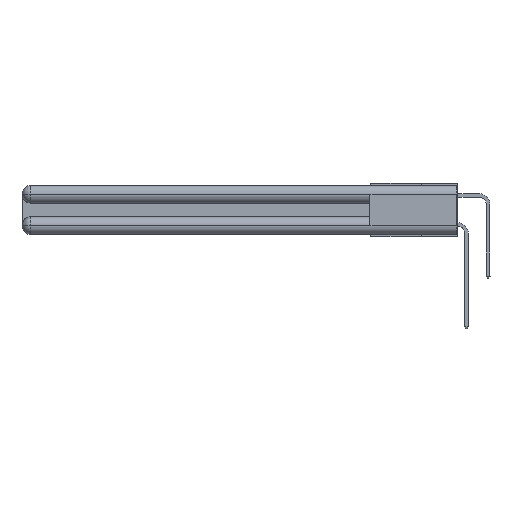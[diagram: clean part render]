
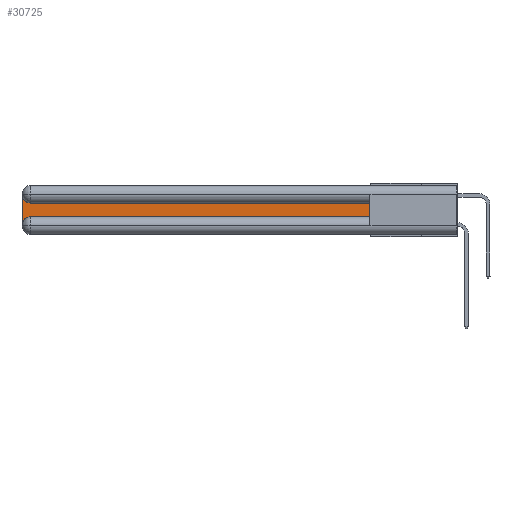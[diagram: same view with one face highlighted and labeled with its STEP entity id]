
A CAD part, left-side view. The second image highlights one B-rep face of the part: STEP entity #30725.
In plain terms, the highlighted planar face has unit normal (-1, 0, 0).
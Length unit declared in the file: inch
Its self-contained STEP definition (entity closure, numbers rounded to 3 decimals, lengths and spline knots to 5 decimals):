
#1558 = DIRECTION ( 'NONE',  ( 0., 0., -1. ) ) ;
#1904 = ORIENTED_EDGE ( 'NONE', *, *, #14672, .T. ) ;
#4491 = EDGE_CURVE ( 'NONE', #7357, #9048, #24010, .T. ) ;
#4784 = VERTEX_POINT ( 'NONE', #15429 ) ;
#5152 = CARTESIAN_POINT ( 'NONE',  ( 0.075, 2.94, -0.2175 ) ) ;
#6355 = CARTESIAN_POINT ( 'NONE',  ( 0.075, 0.6, -0.1225 ) ) ;
#7306 = VERTEX_POINT ( 'NONE', #11868 ) ;
#7357 = VERTEX_POINT ( 'NONE', #20676 ) ;
#7425 = CARTESIAN_POINT ( 'NONE',  ( 0.075, 0.6, -0.2175 ) ) ;
#9048 = VERTEX_POINT ( 'NONE', #22909 ) ;
#9206 = CIRCLE ( 'NONE', #30263, 0.06 ) ;
#9302 = VECTOR ( 'NONE', #30514, 39.37008 ) ;
#9715 = ORIENTED_EDGE ( 'NONE', *, *, #17994, .T. ) ;
#10100 = CIRCLE ( 'NONE', #18869, 0.06 ) ;
#10971 = CARTESIAN_POINT ( 'NONE',  ( 0.075, 2.94, -0.0625 ) ) ;
#11422 = EDGE_CURVE ( 'NONE', #17900, #4784, #22611, .T. ) ;
#11697 = CARTESIAN_POINT ( 'NONE',  ( 0.075, 0.6, -0.2175 ) ) ;
#11840 = DIRECTION ( 'NONE',  ( 0., 0., -1. ) ) ;
#11868 = CARTESIAN_POINT ( 'NONE',  ( 0.075, 0.6, -0.2175 ) ) ;
#12144 = CARTESIAN_POINT ( 'NONE',  ( 0.075, 2.94, -0.2775 ) ) ;
#13028 = VERTEX_POINT ( 'NONE', #5152 ) ;
#13158 = FACE_OUTER_BOUND ( 'NONE', #29761, .T. ) ;
#13498 = DIRECTION ( 'NONE',  ( 0., 0., -1. ) ) ;
#14672 = EDGE_CURVE ( 'NONE', #13028, #7306, #17130, .T. ) ;
#15429 = CARTESIAN_POINT ( 'NONE',  ( 0.075, 2.94, -0.1225 ) ) ;
#16674 = VECTOR ( 'NONE', #11840, 39.37008 ) ;
#17007 = CARTESIAN_POINT ( 'NONE',  ( 0.075, 3., -0.2175 ) ) ;
#17130 = LINE ( 'NONE', #11697, #25758 ) ;
#17900 = VERTEX_POINT ( 'NONE', #6355 ) ;
#17994 = EDGE_CURVE ( 'NONE', #9048, #13028, #9206, .T. ) ;
#18511 = DIRECTION ( 'NONE',  ( 0., 0., 1. ) ) ;
#18869 = AXIS2_PLACEMENT_3D ( 'NONE', #10971, #21700, #13498 ) ;
#20676 = CARTESIAN_POINT ( 'NONE',  ( 0.075, 3., -0.0625 ) ) ;
#21182 = ORIENTED_EDGE ( 'NONE', *, *, #4491, .T. ) ;
#21700 = DIRECTION ( 'NONE',  ( 1., 0., 0. ) ) ;
#22611 = LINE ( 'NONE', #25327, #9302 ) ;
#22909 = CARTESIAN_POINT ( 'NONE',  ( 0.075, 3., -0.2775 ) ) ;
#23523 = LINE ( 'NONE', #7425, #26594 ) ;
#24010 = LINE ( 'NONE', #17007, #16674 ) ;
#25269 = EDGE_CURVE ( 'NONE', #4784, #7357, #10100, .T. ) ;
#25327 = CARTESIAN_POINT ( 'NONE',  ( 0.075, 0.6, -0.1225 ) ) ;
#25758 = VECTOR ( 'NONE', #28194, 39.37008 ) ;
#25883 = ORIENTED_EDGE ( 'NONE', *, *, #11422, .T. ) ;
#25992 = DIRECTION ( 'NONE',  ( 0., 0., -1. ) ) ;
#26515 = CARTESIAN_POINT ( 'NONE',  ( 0.075, 3., -0.1225 ) ) ;
#26594 = VECTOR ( 'NONE', #18511, 39.37008 ) ;
#28194 = DIRECTION ( 'NONE',  ( 0., -1., 0. ) ) ;
#28783 = DIRECTION ( 'NONE',  ( 1., 0., 0. ) ) ;
#29761 = EDGE_LOOP ( 'NONE', ( #25883, #35152, #21182, #9715, #1904, #30460 ) ) ;
#30263 = AXIS2_PLACEMENT_3D ( 'NONE', #12144, #31431, #25992 ) ;
#30460 = ORIENTED_EDGE ( 'NONE', *, *, #33055, .T. ) ;
#30514 = DIRECTION ( 'NONE',  ( 0., 1., 0. ) ) ;
#30725 = ADVANCED_FACE ( 'NONE', ( #13158 ), #31578, .F. ) ;
#31241 = AXIS2_PLACEMENT_3D ( 'NONE', #26515, #28783, #1558 ) ;
#31431 = DIRECTION ( 'NONE',  ( 1., 0., 0. ) ) ;
#31578 = PLANE ( 'NONE',  #31241 ) ;
#33055 = EDGE_CURVE ( 'NONE', #7306, #17900, #23523, .T. ) ;
#35152 = ORIENTED_EDGE ( 'NONE', *, *, #25269, .T. ) ;
